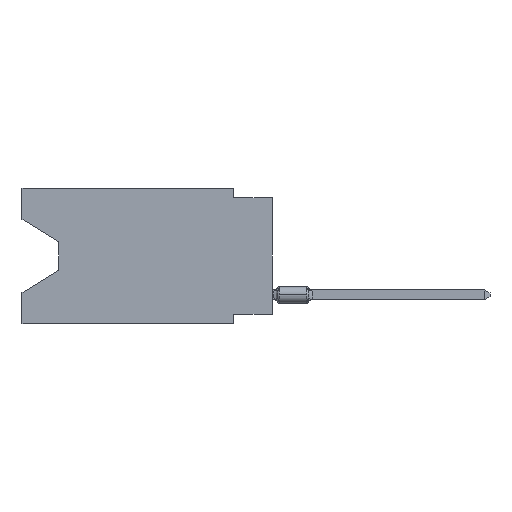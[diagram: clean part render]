
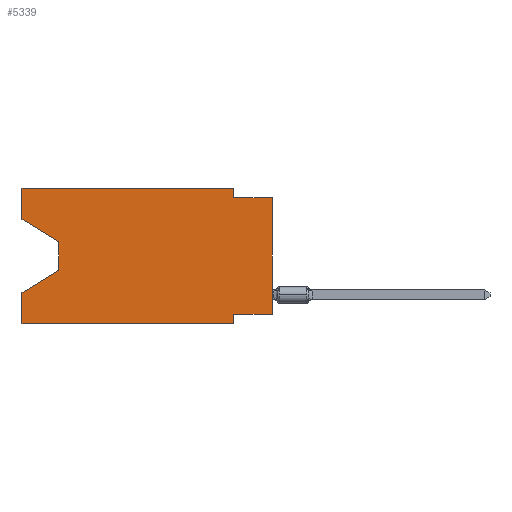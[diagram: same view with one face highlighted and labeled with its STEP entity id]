
A CAD part, left-side view. The second image highlights one B-rep face of the part: STEP entity #5339.
In plain terms, the highlighted planar face has unit normal (-1, 0, 0).
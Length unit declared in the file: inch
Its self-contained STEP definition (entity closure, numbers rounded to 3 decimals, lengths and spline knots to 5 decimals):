
#18 = CARTESIAN_POINT ( 'NONE',  ( 0., 0.645, -0.08025 ) ) ;
#128 = DIRECTION ( 'NONE',  ( 0., 0., -1. ) ) ;
#155 = ORIENTED_EDGE ( 'NONE', *, *, #749, .T. ) ;
#276 = DIRECTION ( 'NONE',  ( 0., -1., 0. ) ) ;
#537 = EDGE_CURVE ( 'NONE', #14477, #4739, #4586, .T. ) ;
#583 = CARTESIAN_POINT ( 'NONE',  ( 0., 0.55, -0.138 ) ) ;
#671 = VERTEX_POINT ( 'NONE', #3828 ) ;
#749 = EDGE_CURVE ( 'NONE', #13491, #11988, #1475, .T. ) ;
#808 = VECTOR ( 'NONE', #4526, 39.37008 ) ;
#830 = CARTESIAN_POINT ( 'NONE',  ( 0., 0.645, 0. ) ) ;
#915 = VECTOR ( 'NONE', #128, 39.37008 ) ;
#1021 = ORIENTED_EDGE ( 'NONE', *, *, #4233, .T. ) ;
#1051 = VERTEX_POINT ( 'NONE', #6767 ) ;
#1193 = CARTESIAN_POINT ( 'NONE',  ( 0., 0., -0.025 ) ) ;
#1316 = CARTESIAN_POINT ( 'NONE',  ( 0., 0.645, -0.08025 ) ) ;
#1349 = LINE ( 'NONE', #3468, #915 ) ;
#1475 = LINE ( 'NONE', #1316, #4216 ) ;
#1877 = DIRECTION ( 'NONE',  ( 0., 0., -1. ) ) ;
#1907 = LINE ( 'NONE', #6384, #5918 ) ;
#2121 = CARTESIAN_POINT ( 'NONE',  ( 0., 0.645, 0. ) ) ;
#2721 = ORIENTED_EDGE ( 'NONE', *, *, #12501, .F. ) ;
#2799 = ORIENTED_EDGE ( 'NONE', *, *, #14881, .T. ) ;
#2837 = VECTOR ( 'NONE', #6462, 39.37008 ) ;
#2847 = LINE ( 'NONE', #13338, #14026 ) ;
#2914 = ORIENTED_EDGE ( 'NONE', *, *, #11323, .F. ) ;
#2915 = VERTEX_POINT ( 'NONE', #6511 ) ;
#2932 = ORIENTED_EDGE ( 'NONE', *, *, #10029, .T. ) ;
#3045 = DIRECTION ( 'NONE',  ( 0., 0., -1. ) ) ;
#3468 = CARTESIAN_POINT ( 'NONE',  ( 0., 0.1, -0.35 ) ) ;
#3699 = EDGE_CURVE ( 'NONE', #12699, #5519, #11112, .T. ) ;
#3798 = CARTESIAN_POINT ( 'NONE',  ( 0., 0., -0.325 ) ) ;
#3828 = CARTESIAN_POINT ( 'NONE',  ( 0., 0.645, 0. ) ) ;
#4216 = VECTOR ( 'NONE', #10737, 39.37008 ) ;
#4233 = EDGE_CURVE ( 'NONE', #10140, #4739, #11682, .T. ) ;
#4526 = DIRECTION ( 'NONE',  ( 0., 0.855, -0.519 ) ) ;
#4586 = LINE ( 'NONE', #5713, #6637 ) ;
#4739 = VERTEX_POINT ( 'NONE', #10669 ) ;
#4868 = ORIENTED_EDGE ( 'NONE', *, *, #13259, .F. ) ;
#5339 = ADVANCED_FACE ( 'NONE', ( #14662 ), #13527, .F. ) ;
#5371 = EDGE_CURVE ( 'NONE', #671, #7004, #8047, .T. ) ;
#5519 = VERTEX_POINT ( 'NONE', #6135 ) ;
#5713 = CARTESIAN_POINT ( 'NONE',  ( 0., 0.645, 0. ) ) ;
#5914 = EDGE_CURVE ( 'NONE', #2915, #5519, #8099, .T. ) ;
#5918 = VECTOR ( 'NONE', #3045, 39.37008 ) ;
#6135 = CARTESIAN_POINT ( 'NONE',  ( 0., 0., -0.025 ) ) ;
#6156 = VECTOR ( 'NONE', #9098, 39.37008 ) ;
#6194 = AXIS2_PLACEMENT_3D ( 'NONE', #830, #14822, #7980 ) ;
#6228 = VECTOR ( 'NONE', #1877, 39.37008 ) ;
#6339 = DIRECTION ( 'NONE',  ( 0., 1., 0. ) ) ;
#6384 = CARTESIAN_POINT ( 'NONE',  ( 0., 0.1, 0. ) ) ;
#6462 = DIRECTION ( 'NONE',  ( 0., 0., 1. ) ) ;
#6511 = CARTESIAN_POINT ( 'NONE',  ( 0., 0.1, -0.025 ) ) ;
#6637 = VECTOR ( 'NONE', #10357, 39.37008 ) ;
#6727 = VERTEX_POINT ( 'NONE', #14533 ) ;
#6767 = CARTESIAN_POINT ( 'NONE',  ( 0., 0.1, -0.35 ) ) ;
#6805 = CARTESIAN_POINT ( 'NONE',  ( 0., 0.55, -0.212 ) ) ;
#7004 = VERTEX_POINT ( 'NONE', #14897 ) ;
#7221 = VECTOR ( 'NONE', #14388, 39.37008 ) ;
#7828 = LINE ( 'NONE', #14599, #2837 ) ;
#7902 = EDGE_CURVE ( 'NONE', #7004, #2915, #1907, .T. ) ;
#7980 = DIRECTION ( 'NONE',  ( 0., 0., -1. ) ) ;
#8047 = LINE ( 'NONE', #2121, #6156 ) ;
#8099 = LINE ( 'NONE', #1193, #14004 ) ;
#8479 = CARTESIAN_POINT ( 'NONE',  ( 0., 0.55, -0.138 ) ) ;
#8792 = LINE ( 'NONE', #12099, #12852 ) ;
#8990 = ORIENTED_EDGE ( 'NONE', *, *, #5371, .F. ) ;
#9098 = DIRECTION ( 'NONE',  ( 0., -1., 0. ) ) ;
#9867 = DIRECTION ( 'NONE',  ( 0., -1., 0. ) ) ;
#10029 = EDGE_CURVE ( 'NONE', #11988, #10140, #14426, .T. ) ;
#10140 = VERTEX_POINT ( 'NONE', #6805 ) ;
#10357 = DIRECTION ( 'NONE',  ( 0., 0., 1. ) ) ;
#10532 = ORIENTED_EDGE ( 'NONE', *, *, #3699, .T. ) ;
#10669 = CARTESIAN_POINT ( 'NONE',  ( 0., 0.645, -0.26975 ) ) ;
#10737 = DIRECTION ( 'NONE',  ( 0., -0.855, -0.519 ) ) ;
#10894 = CARTESIAN_POINT ( 'NONE',  ( 0., 0., 0. ) ) ;
#11112 = LINE ( 'NONE', #10894, #7221 ) ;
#11323 = EDGE_CURVE ( 'NONE', #6727, #1051, #1349, .T. ) ;
#11682 = LINE ( 'NONE', #15031, #808 ) ;
#11865 = ORIENTED_EDGE ( 'NONE', *, *, #5914, .F. ) ;
#11977 = CARTESIAN_POINT ( 'NONE',  ( 0., 0.645, -0.35 ) ) ;
#11988 = VERTEX_POINT ( 'NONE', #8479 ) ;
#12099 = CARTESIAN_POINT ( 'NONE',  ( 0., 0.645, -0.35 ) ) ;
#12159 = ORIENTED_EDGE ( 'NONE', *, *, #7902, .F. ) ;
#12501 = EDGE_CURVE ( 'NONE', #13491, #671, #7828, .T. ) ;
#12699 = VERTEX_POINT ( 'NONE', #3798 ) ;
#12852 = VECTOR ( 'NONE', #9867, 39.37008 ) ;
#13138 = EDGE_LOOP ( 'NONE', ( #155, #2932, #1021, #14766, #2799, #2914, #4868, #10532, #11865, #12159, #8990, #2721 ) ) ;
#13259 = EDGE_CURVE ( 'NONE', #12699, #6727, #2847, .T. ) ;
#13338 = CARTESIAN_POINT ( 'NONE',  ( 0., 0., -0.325 ) ) ;
#13491 = VERTEX_POINT ( 'NONE', #18 ) ;
#13527 = PLANE ( 'NONE',  #6194 ) ;
#14004 = VECTOR ( 'NONE', #276, 39.37008 ) ;
#14026 = VECTOR ( 'NONE', #6339, 39.37008 ) ;
#14388 = DIRECTION ( 'NONE',  ( 0., 0., 1. ) ) ;
#14426 = LINE ( 'NONE', #583, #6228 ) ;
#14477 = VERTEX_POINT ( 'NONE', #11977 ) ;
#14533 = CARTESIAN_POINT ( 'NONE',  ( 0., 0.1, -0.325 ) ) ;
#14599 = CARTESIAN_POINT ( 'NONE',  ( 0., 0.645, 0. ) ) ;
#14662 = FACE_OUTER_BOUND ( 'NONE', #13138, .T. ) ;
#14766 = ORIENTED_EDGE ( 'NONE', *, *, #537, .F. ) ;
#14822 = DIRECTION ( 'NONE',  ( 1., 0., 0. ) ) ;
#14881 = EDGE_CURVE ( 'NONE', #14477, #1051, #8792, .T. ) ;
#14897 = CARTESIAN_POINT ( 'NONE',  ( 0., 0.1, 0. ) ) ;
#15031 = CARTESIAN_POINT ( 'NONE',  ( 0., 0.55, -0.212 ) ) ;
